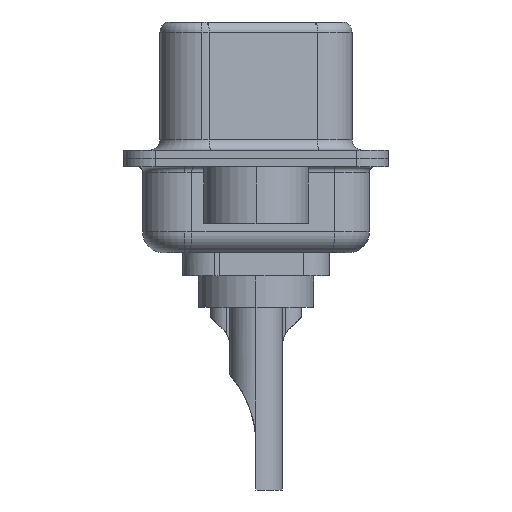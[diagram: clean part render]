
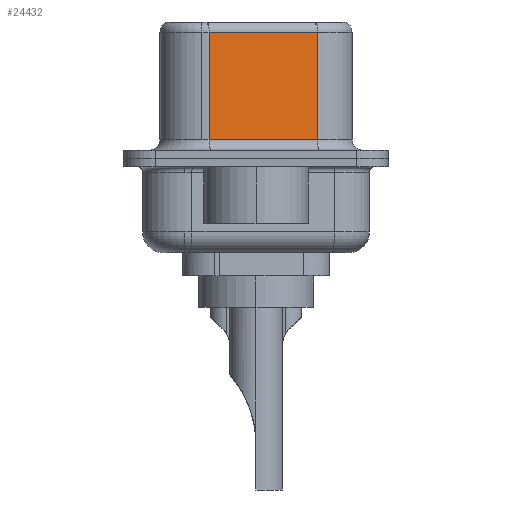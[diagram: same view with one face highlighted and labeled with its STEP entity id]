
A CAD part, left-side view. The second image highlights one B-rep face of the part: STEP entity #24432.
In plain terms, the highlighted planar face has unit normal (-0.985, -0.174, 0).
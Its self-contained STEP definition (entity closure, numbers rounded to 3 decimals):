
#55 = ORIENTED_EDGE ( 'NONE', *, *, #19802, .T. ) ;
#266 = CARTESIAN_POINT ( 'NONE',  ( 3.67, 2.233, 6.02 ) ) ;
#677 = ORIENTED_EDGE ( 'NONE', *, *, #15353, .T. ) ;
#865 = ORIENTED_EDGE ( 'NONE', *, *, #4245, .T. ) ;
#1238 = LINE ( 'NONE', #21246, #7495 ) ;
#2838 = EDGE_CURVE ( 'NONE', #23773, #10558, #23785, .T. ) ;
#4245 = EDGE_CURVE ( 'NONE', #13134, #10558, #10879, .T. ) ;
#6147 = CARTESIAN_POINT ( 'NONE',  ( 3.67, 2.233, 0.9 ) ) ;
#6886 = CARTESIAN_POINT ( 'NONE',  ( 4.58, -2.927, 6.52 ) ) ;
#7047 = CARTESIAN_POINT ( 'NONE',  ( 4.58, -2.927, 0.9 ) ) ;
#7065 = AXIS2_PLACEMENT_3D ( 'NONE', #6886, #8933, #22983 ) ;
#7355 = VECTOR ( 'NONE', #7928, 1000. ) ;
#7495 = VECTOR ( 'NONE', #11248, 1000. ) ;
#7928 = DIRECTION ( 'NONE',  ( 0., 0., -1. ) ) ;
#8669 = VECTOR ( 'NONE', #9932, 1000. ) ;
#8853 = PLANE ( 'NONE',  #7065 ) ;
#8933 = DIRECTION ( 'NONE',  ( 0.985, 0.174, 0. ) ) ;
#9750 = VERTEX_POINT ( 'NONE', #266 ) ;
#9932 = DIRECTION ( 'NONE',  ( 0., 0., -1. ) ) ;
#10558 = VERTEX_POINT ( 'NONE', #7047 ) ;
#10808 = CARTESIAN_POINT ( 'NONE',  ( 4.58, -2.927, 6.52 ) ) ;
#10879 = LINE ( 'NONE', #23781, #26175 ) ;
#11248 = DIRECTION ( 'NONE',  ( -0.174, 0.985, 0. ) ) ;
#13134 = VERTEX_POINT ( 'NONE', #6147 ) ;
#15134 = EDGE_LOOP ( 'NONE', ( #16602, #55, #677, #865 ) ) ;
#15353 = EDGE_CURVE ( 'NONE', #9750, #13134, #23406, .T. ) ;
#16602 = ORIENTED_EDGE ( 'NONE', *, *, #2838, .F. ) ;
#16841 = DIRECTION ( 'NONE',  ( 0.174, -0.985, 0. ) ) ;
#18079 = CARTESIAN_POINT ( 'NONE',  ( 3.67, 2.233, 6.52 ) ) ;
#19537 = FACE_OUTER_BOUND ( 'NONE', #15134, .T. ) ;
#19802 = EDGE_CURVE ( 'NONE', #23773, #9750, #1238, .T. ) ;
#20955 = CARTESIAN_POINT ( 'NONE',  ( 4.58, -2.927, 6.02 ) ) ;
#21246 = CARTESIAN_POINT ( 'NONE',  ( 4.58, -2.927, 6.02 ) ) ;
#22983 = DIRECTION ( 'NONE',  ( -0.174, 0.985, 0. ) ) ;
#23406 = LINE ( 'NONE', #18079, #7355 ) ;
#23773 = VERTEX_POINT ( 'NONE', #20955 ) ;
#23781 = CARTESIAN_POINT ( 'NONE',  ( 4.58, -2.927, 0.9 ) ) ;
#23785 = LINE ( 'NONE', #10808, #8669 ) ;
#24432 = ADVANCED_FACE ( 'NONE', ( #19537 ), #8853, .F. ) ;
#26175 = VECTOR ( 'NONE', #16841, 1000. ) ;
